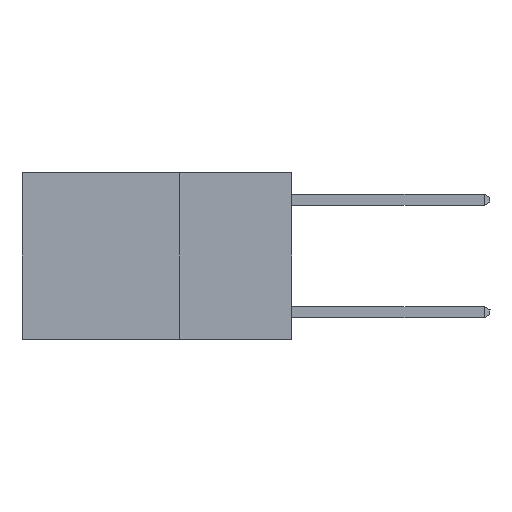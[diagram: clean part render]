
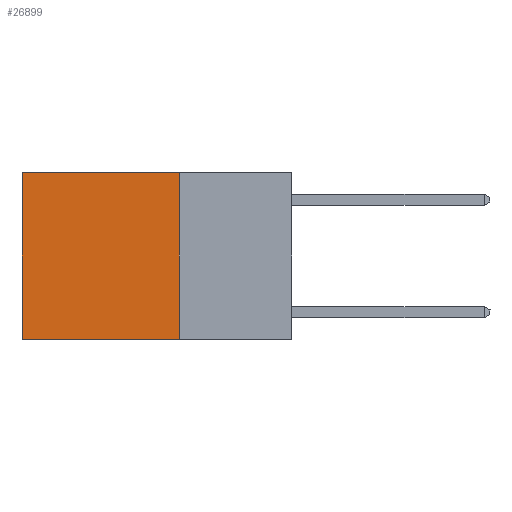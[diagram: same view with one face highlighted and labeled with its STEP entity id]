
A CAD part, left-side view. The second image highlights one B-rep face of the part: STEP entity #26899.
In plain terms, the highlighted planar face has unit normal (-1, 0, 0).
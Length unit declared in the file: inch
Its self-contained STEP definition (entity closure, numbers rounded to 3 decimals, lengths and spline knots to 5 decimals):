
#317 = DIRECTION ( 'NONE',  ( 0., 1., 0. ) ) ;
#367 = CARTESIAN_POINT ( 'NONE',  ( 0.2625, 0.25, 0. ) ) ;
#397 = LINE ( 'NONE', #26475, #5404 ) ;
#779 = DIRECTION ( 'NONE',  ( 0., 0., -1. ) ) ;
#1030 = EDGE_CURVE ( 'NONE', #15941, #9927, #397, .T. ) ;
#2667 = CARTESIAN_POINT ( 'NONE',  ( 0.2625, 0.6, 0. ) ) ;
#5404 = VECTOR ( 'NONE', #20318, 39.37008 ) ;
#7104 = CARTESIAN_POINT ( 'NONE',  ( 0.2625, 0.25, 0. ) ) ;
#8001 = ORIENTED_EDGE ( 'NONE', *, *, #1030, .F. ) ;
#8665 = EDGE_CURVE ( 'NONE', #13014, #22155, #21577, .T. ) ;
#9387 = DIRECTION ( 'NONE',  ( 0., 0., -1. ) ) ;
#9927 = VERTEX_POINT ( 'NONE', #11250 ) ;
#9969 = ORIENTED_EDGE ( 'NONE', *, *, #22535, .T. ) ;
#11250 = CARTESIAN_POINT ( 'NONE',  ( 0.2625, 0.25, -0.37 ) ) ;
#11394 = CARTESIAN_POINT ( 'NONE',  ( 0.2625, 0.6, 0. ) ) ;
#12679 = CARTESIAN_POINT ( 'NONE',  ( 0.2625, 0.6, -0.37 ) ) ;
#12933 = CARTESIAN_POINT ( 'NONE',  ( 0.2625, 0.25, -0.37 ) ) ;
#13014 = VERTEX_POINT ( 'NONE', #2667 ) ;
#13416 = DIRECTION ( 'NONE',  ( 1., 0., 0. ) ) ;
#13743 = ORIENTED_EDGE ( 'NONE', *, *, #8665, .T. ) ;
#13769 = DIRECTION ( 'NONE',  ( 0., 1., 0. ) ) ;
#14351 = VECTOR ( 'NONE', #317, 39.37008 ) ;
#14715 = LINE ( 'NONE', #24164, #25111 ) ;
#15941 = VERTEX_POINT ( 'NONE', #367 ) ;
#16068 = VECTOR ( 'NONE', #9387, 39.37008 ) ;
#17044 = FACE_OUTER_BOUND ( 'NONE', #17165, .T. ) ;
#17165 = EDGE_LOOP ( 'NONE', ( #13743, #19234, #8001, #9969 ) ) ;
#18626 = LINE ( 'NONE', #12933, #14351 ) ;
#19234 = ORIENTED_EDGE ( 'NONE', *, *, #22816, .F. ) ;
#20318 = DIRECTION ( 'NONE',  ( 0., 0., -1. ) ) ;
#21577 = LINE ( 'NONE', #11394, #16068 ) ;
#22155 = VERTEX_POINT ( 'NONE', #12679 ) ;
#22535 = EDGE_CURVE ( 'NONE', #15941, #13014, #14715, .T. ) ;
#22816 = EDGE_CURVE ( 'NONE', #9927, #22155, #18626, .T. ) ;
#24164 = CARTESIAN_POINT ( 'NONE',  ( 0.2625, 0.25, 0. ) ) ;
#25111 = VECTOR ( 'NONE', #13769, 39.37008 ) ;
#25402 = AXIS2_PLACEMENT_3D ( 'NONE', #7104, #13416, #779 ) ;
#25888 = PLANE ( 'NONE',  #25402 ) ;
#26475 = CARTESIAN_POINT ( 'NONE',  ( 0.2625, 0.25, 0. ) ) ;
#26899 = ADVANCED_FACE ( 'NONE', ( #17044 ), #25888, .F. ) ;
